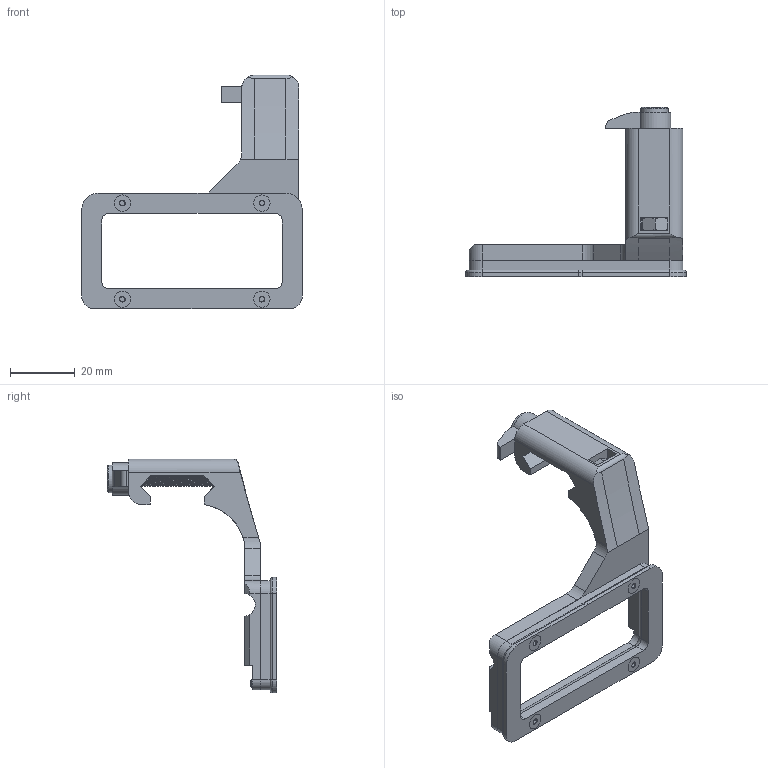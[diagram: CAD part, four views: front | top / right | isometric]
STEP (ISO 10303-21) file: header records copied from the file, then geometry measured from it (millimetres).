
FILE_DESCRIPTION(/* description */ (''),/* implementation_level */ '2;1');
FILE_NAME(/* name */ 'SOCK BRASS CATCHER.stp',/* time_stamp */ '2020-10-20T18:14:12+03:00',/* author */ (''),/* organization */ (''),/* preprocessor_version */ 'ST-DEVELOPER v15.2',/* originating_system */ 'Autodesk Translator Framework v2.0.0.5431',/* authorisation */ '');
FILE_SCHEMA (('AUTOMOTIVE_DESIGN { 1 0 10303 214 3 1 1 }'));
Products named in the file (1): SOCK BRASS CATCHER
Bounding box: 67.86 x 52.1 x 72 mm (x, y, z)
Volume: 16319.1 mm3; surface area: 13287.1 mm2
Topology: 9 solids, 9 shells, 346 faces, 1303 edges, 978 vertices
Faces by surface type: cylinder 126, plane 124, cone 64, bspline 24, torus 8
Full cylindrical faces by diameter (mm): 2.5 x4, 5 x53, 8.5 x2
Entity records: 36002 total; most frequent: CARTESIAN_POINT 26859, ORIENTED_EDGE 2426, DIRECTION 1318, EDGE_CURVE 1213, VERTEX_POINT 968, AXIS2_PLACEMENT_3D 520, B_SPLINE_CURVE_WITH_KNOTS 519, EDGE_LOOP 371
